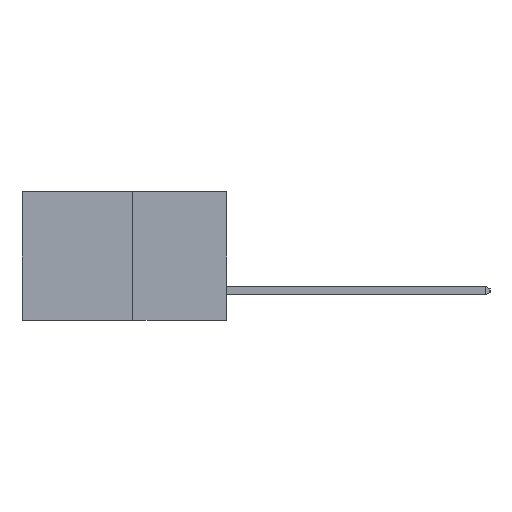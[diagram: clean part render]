
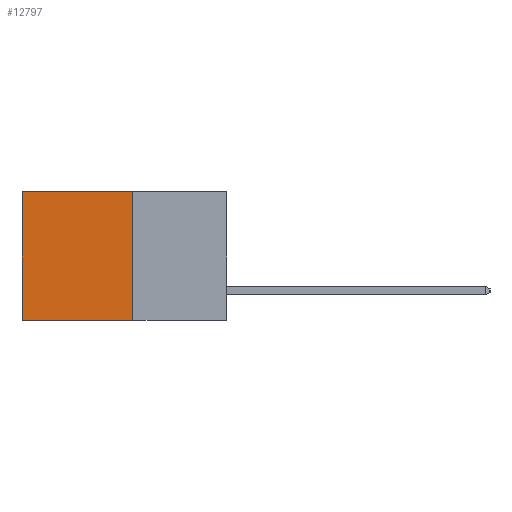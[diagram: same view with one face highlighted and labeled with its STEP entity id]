
A CAD part, left-side view. The second image highlights one B-rep face of the part: STEP entity #12797.
In plain terms, the highlighted planar face has unit normal (-1, 0, 0).
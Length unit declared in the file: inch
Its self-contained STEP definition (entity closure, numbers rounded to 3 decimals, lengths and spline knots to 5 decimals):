
#120 = CARTESIAN_POINT ( 'NONE',  ( 0.277, 0.27, -0.37 ) ) ;
#276 = LINE ( 'NONE', #3612, #5600 ) ;
#517 = EDGE_LOOP ( 'NONE', ( #12790, #11328, #8081, #7920 ) ) ;
#1214 = DIRECTION ( 'NONE',  ( 0., 0., -1. ) ) ;
#1482 = EDGE_CURVE ( 'NONE', #3816, #4976, #12218, .T. ) ;
#1614 = CARTESIAN_POINT ( 'NONE',  ( 0.277, 0.27, -0.37 ) ) ;
#2120 = EDGE_CURVE ( 'NONE', #3816, #8816, #12539, .T. ) ;
#2914 = LINE ( 'NONE', #1614, #11071 ) ;
#3050 = CARTESIAN_POINT ( 'NONE',  ( 0.277, 0.27, 0. ) ) ;
#3583 = DIRECTION ( 'NONE',  ( 0., 0., -1. ) ) ;
#3612 = CARTESIAN_POINT ( 'NONE',  ( 0.277, 0.59, -0.37 ) ) ;
#3816 = VERTEX_POINT ( 'NONE', #3050 ) ;
#4343 = PLANE ( 'NONE',  #10679 ) ;
#4976 = VERTEX_POINT ( 'NONE', #9872 ) ;
#5600 = VECTOR ( 'NONE', #3583, 39.37008 ) ;
#7359 = FACE_OUTER_BOUND ( 'NONE', #517, .T. ) ;
#7460 = DIRECTION ( 'NONE',  ( 1., 0., 0. ) ) ;
#7635 = VERTEX_POINT ( 'NONE', #8527 ) ;
#7828 = DIRECTION ( 'NONE',  ( 0., 1., 0. ) ) ;
#7920 = ORIENTED_EDGE ( 'NONE', *, *, #1482, .T. ) ;
#8081 = ORIENTED_EDGE ( 'NONE', *, *, #2120, .F. ) ;
#8169 = EDGE_CURVE ( 'NONE', #4976, #7635, #276, .T. ) ;
#8527 = CARTESIAN_POINT ( 'NONE',  ( 0.277, 0.59, -0.37 ) ) ;
#8747 = DIRECTION ( 'NONE',  ( 0., 1., 0. ) ) ;
#8816 = VERTEX_POINT ( 'NONE', #8822 ) ;
#8822 = CARTESIAN_POINT ( 'NONE',  ( 0.277, 0.27, -0.37 ) ) ;
#8842 = EDGE_CURVE ( 'NONE', #8816, #7635, #2914, .T. ) ;
#9872 = CARTESIAN_POINT ( 'NONE',  ( 0.277, 0.59, 0. ) ) ;
#10679 = AXIS2_PLACEMENT_3D ( 'NONE', #120, #7460, #1214 ) ;
#11071 = VECTOR ( 'NONE', #7828, 39.37008 ) ;
#11328 = ORIENTED_EDGE ( 'NONE', *, *, #8842, .F. ) ;
#11923 = VECTOR ( 'NONE', #8747, 39.37008 ) ;
#12215 = CARTESIAN_POINT ( 'NONE',  ( 0.277, 0.27, 0. ) ) ;
#12218 = LINE ( 'NONE', #12215, #11923 ) ;
#12291 = CARTESIAN_POINT ( 'NONE',  ( 0.277, 0.27, -0.37 ) ) ;
#12539 = LINE ( 'NONE', #12291, #12835 ) ;
#12790 = ORIENTED_EDGE ( 'NONE', *, *, #8169, .T. ) ;
#12797 = ADVANCED_FACE ( 'NONE', ( #7359 ), #4343, .F. ) ;
#12835 = VECTOR ( 'NONE', #13002, 39.37008 ) ;
#13002 = DIRECTION ( 'NONE',  ( 0., 0., -1. ) ) ;
